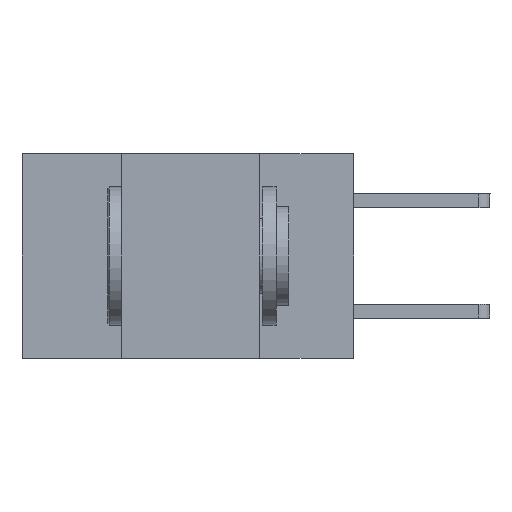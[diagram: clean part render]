
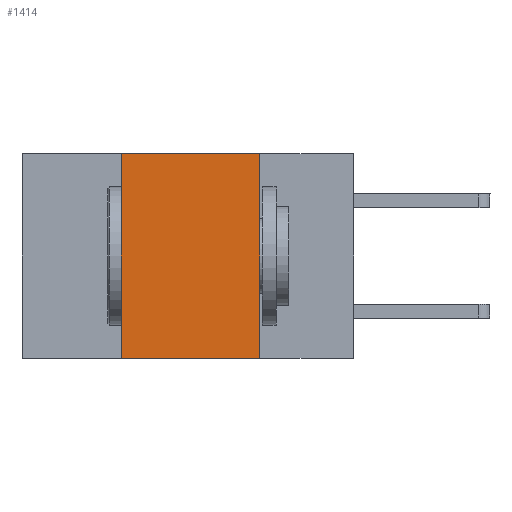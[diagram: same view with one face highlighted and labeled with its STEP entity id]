
A CAD part, left-side view. The second image highlights one B-rep face of the part: STEP entity #1414.
In plain terms, the highlighted planar face has unit normal (-1, 0, 0).
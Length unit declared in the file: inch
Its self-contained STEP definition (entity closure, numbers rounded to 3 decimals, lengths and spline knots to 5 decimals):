
#198 = CARTESIAN_POINT ( 'NONE',  ( 0., 0.6, -0.37 ) ) ;
#612 = LINE ( 'NONE', #9558, #2291 ) ;
#851 = LINE ( 'NONE', #10981, #11749 ) ;
#1012 = DIRECTION ( 'NONE',  ( 0., 0., -1. ) ) ;
#1058 = VERTEX_POINT ( 'NONE', #4285 ) ;
#1084 = CARTESIAN_POINT ( 'NONE',  ( 0., 0.42, 0. ) ) ;
#1397 = VERTEX_POINT ( 'NONE', #3790 ) ;
#1414 = ADVANCED_FACE ( 'NONE', ( #2948 ), #6946, .F. ) ;
#1589 = DIRECTION ( 'NONE',  ( 0., -1., 0. ) ) ;
#1975 = CARTESIAN_POINT ( 'NONE',  ( 0., 0.6, 0. ) ) ;
#2075 = DIRECTION ( 'NONE',  ( 0., 0., -1. ) ) ;
#2291 = VECTOR ( 'NONE', #1589, 39.37008 ) ;
#2502 = ORIENTED_EDGE ( 'NONE', *, *, #12319, .F. ) ;
#2948 = FACE_OUTER_BOUND ( 'NONE', #10621, .T. ) ;
#2957 = VECTOR ( 'NONE', #9581, 39.37008 ) ;
#3790 = CARTESIAN_POINT ( 'NONE',  ( 0., 0.17, 0. ) ) ;
#4285 = CARTESIAN_POINT ( 'NONE',  ( 0., 0.17, -0.37 ) ) ;
#4327 = ORIENTED_EDGE ( 'NONE', *, *, #6296, .F. ) ;
#4558 = ORIENTED_EDGE ( 'NONE', *, *, #9753, .F. ) ;
#5591 = CARTESIAN_POINT ( 'NONE',  ( 0., 0.42, 0. ) ) ;
#5610 = AXIS2_PLACEMENT_3D ( 'NONE', #1975, #5972, #1012 ) ;
#5972 = DIRECTION ( 'NONE',  ( 1., 0., 0. ) ) ;
#6296 = EDGE_CURVE ( 'NONE', #9891, #1397, #612, .T. ) ;
#6946 = PLANE ( 'NONE',  #5610 ) ;
#8655 = ORIENTED_EDGE ( 'NONE', *, *, #9324, .T. ) ;
#8953 = DIRECTION ( 'NONE',  ( 0., -1., 0. ) ) ;
#9084 = LINE ( 'NONE', #198, #12759 ) ;
#9324 = EDGE_CURVE ( 'NONE', #12185, #1058, #9084, .T. ) ;
#9558 = CARTESIAN_POINT ( 'NONE',  ( 0., 0.6, 0. ) ) ;
#9581 = DIRECTION ( 'NONE',  ( 0., 0., 1. ) ) ;
#9753 = EDGE_CURVE ( 'NONE', #12185, #9891, #12571, .T. ) ;
#9891 = VERTEX_POINT ( 'NONE', #1084 ) ;
#10621 = EDGE_LOOP ( 'NONE', ( #2502, #4327, #4558, #8655 ) ) ;
#10981 = CARTESIAN_POINT ( 'NONE',  ( 0., 0.17, 0. ) ) ;
#11749 = VECTOR ( 'NONE', #2075, 39.37008 ) ;
#11808 = CARTESIAN_POINT ( 'NONE',  ( 0., 0.42, -0.37 ) ) ;
#12185 = VERTEX_POINT ( 'NONE', #11808 ) ;
#12319 = EDGE_CURVE ( 'NONE', #1397, #1058, #851, .T. ) ;
#12571 = LINE ( 'NONE', #5591, #2957 ) ;
#12759 = VECTOR ( 'NONE', #8953, 39.37008 ) ;
